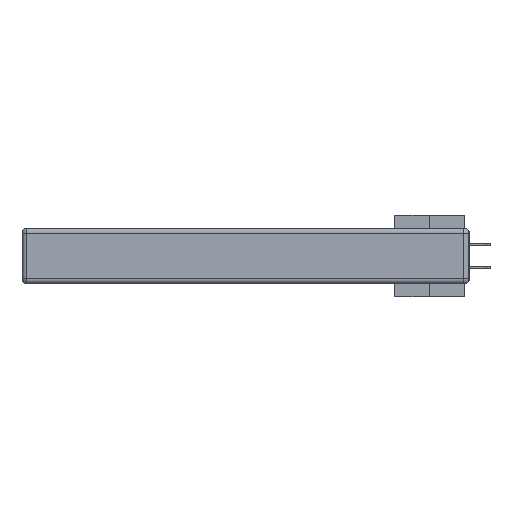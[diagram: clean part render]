
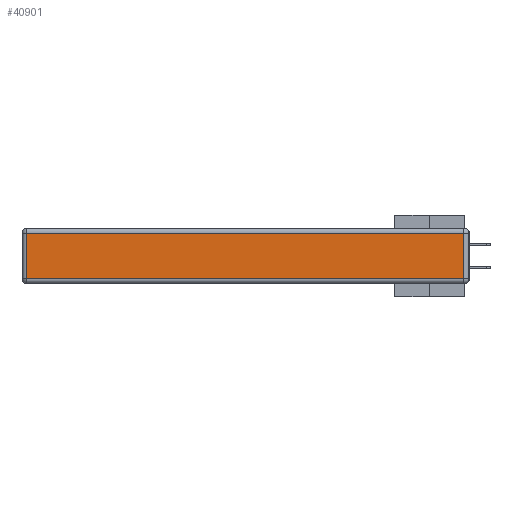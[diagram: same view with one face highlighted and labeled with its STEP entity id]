
A CAD part, left-side view. The second image highlights one B-rep face of the part: STEP entity #40901.
In plain terms, the highlighted planar face has unit normal (-1, 0, 0).
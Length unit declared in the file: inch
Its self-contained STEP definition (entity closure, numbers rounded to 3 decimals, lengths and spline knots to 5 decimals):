
#1428 = CARTESIAN_POINT ( 'NONE',  ( 0., 2.72, -0.03 ) ) ;
#2278 = LINE ( 'NONE', #36241, #12435 ) ;
#3858 = CARTESIAN_POINT ( 'NONE',  ( 0., 0.03, -0.03 ) ) ;
#5420 = VERTEX_POINT ( 'NONE', #43383 ) ;
#5942 = VERTEX_POINT ( 'NONE', #3858 ) ;
#7374 = LINE ( 'NONE', #8412, #25044 ) ;
#8412 = CARTESIAN_POINT ( 'NONE',  ( 0., 2.72, -0.343 ) ) ;
#9763 = EDGE_CURVE ( 'NONE', #20178, #5942, #13632, .T. ) ;
#11751 = LINE ( 'NONE', #14651, #42772 ) ;
#12435 = VECTOR ( 'NONE', #23679, 39.37008 ) ;
#13632 = LINE ( 'NONE', #17044, #35551 ) ;
#14651 = CARTESIAN_POINT ( 'NONE',  ( 0., 0., -0.313 ) ) ;
#14745 = ORIENTED_EDGE ( 'NONE', *, *, #9763, .T. ) ;
#15085 = ORIENTED_EDGE ( 'NONE', *, *, #39663, .T. ) ;
#16190 = DIRECTION ( 'NONE',  ( 0., 0., 1. ) ) ;
#17044 = CARTESIAN_POINT ( 'NONE',  ( 0., 0.03, -0.343 ) ) ;
#17355 = DIRECTION ( 'NONE',  ( 0., 0., 1. ) ) ;
#18307 = EDGE_CURVE ( 'NONE', #5420, #20178, #11751, .T. ) ;
#19259 = AXIS2_PLACEMENT_3D ( 'NONE', #23646, #29799, #16190 ) ;
#19649 = EDGE_CURVE ( 'NONE', #32665, #5420, #7374, .T. ) ;
#20178 = VERTEX_POINT ( 'NONE', #38977 ) ;
#23646 = CARTESIAN_POINT ( 'NONE',  ( 0., 0., -0.343 ) ) ;
#23679 = DIRECTION ( 'NONE',  ( 0., 1., 0. ) ) ;
#25044 = VECTOR ( 'NONE', #35758, 39.37008 ) ;
#29799 = DIRECTION ( 'NONE',  ( -1., 0., 0. ) ) ;
#32665 = VERTEX_POINT ( 'NONE', #1428 ) ;
#35551 = VECTOR ( 'NONE', #17355, 39.37008 ) ;
#35758 = DIRECTION ( 'NONE',  ( 0., 0., -1. ) ) ;
#36241 = CARTESIAN_POINT ( 'NONE',  ( 0., 2.75, -0.03 ) ) ;
#36661 = ORIENTED_EDGE ( 'NONE', *, *, #19649, .T. ) ;
#37388 = EDGE_LOOP ( 'NONE', ( #41463, #14745, #15085, #36661 ) ) ;
#38977 = CARTESIAN_POINT ( 'NONE',  ( 0., 0.03, -0.313 ) ) ;
#39563 = FACE_OUTER_BOUND ( 'NONE', #37388, .T. ) ;
#39663 = EDGE_CURVE ( 'NONE', #5942, #32665, #2278, .T. ) ;
#40654 = PLANE ( 'NONE',  #19259 ) ;
#40901 = ADVANCED_FACE ( 'NONE', ( #39563 ), #40654, .T. ) ;
#41463 = ORIENTED_EDGE ( 'NONE', *, *, #18307, .T. ) ;
#41958 = DIRECTION ( 'NONE',  ( 0., -1., 0. ) ) ;
#42772 = VECTOR ( 'NONE', #41958, 39.37008 ) ;
#43383 = CARTESIAN_POINT ( 'NONE',  ( 0., 2.72, -0.313 ) ) ;
